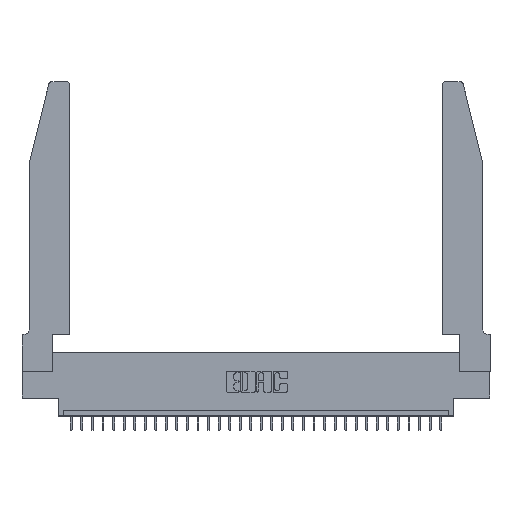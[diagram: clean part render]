
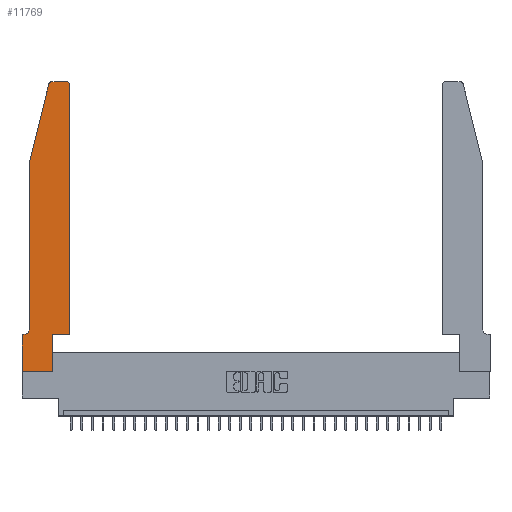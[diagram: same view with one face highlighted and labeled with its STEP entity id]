
A CAD part, top view. The second image highlights one B-rep face of the part: STEP entity #11769.
In plain terms, the highlighted planar face has unit normal (0, 0, 1).
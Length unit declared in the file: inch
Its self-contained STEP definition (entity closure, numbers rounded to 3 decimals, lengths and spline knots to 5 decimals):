
#304 = CARTESIAN_POINT ( 'NONE',  ( 0.284, 2.72, 0.37 ) ) ;
#1247 = PLANE ( 'NONE',  #5234 ) ;
#1288 = ORIENTED_EDGE ( 'NONE', *, *, #5457, .T. ) ;
#1545 = VERTEX_POINT ( 'NONE', #21221 ) ;
#2732 = ORIENTED_EDGE ( 'NONE', *, *, #26370, .T. ) ;
#2851 = LINE ( 'NONE', #30953, #15270 ) ;
#2899 = CARTESIAN_POINT ( 'NONE',  ( 0.4505, 0.35, 0.37 ) ) ;
#3214 = AXIS2_PLACEMENT_3D ( 'NONE', #30243, #17447, #30412 ) ;
#3261 = CARTESIAN_POINT ( 'NONE',  ( 0.2865, 0.35, 0.37 ) ) ;
#3734 = EDGE_CURVE ( 'NONE', #28187, #17740, #19510, .T. ) ;
#3958 = CARTESIAN_POINT ( 'NONE',  ( 0., 0., 0.37 ) ) ;
#4308 = VERTEX_POINT ( 'NONE', #21942 ) ;
#5141 = ORIENTED_EDGE ( 'NONE', *, *, #23761, .T. ) ;
#5234 = AXIS2_PLACEMENT_3D ( 'NONE', #29333, #29814, #16689 ) ;
#5243 = ORIENTED_EDGE ( 'NONE', *, *, #31368, .T. ) ;
#5287 = VERTEX_POINT ( 'NONE', #27833 ) ;
#5293 = DIRECTION ( 'NONE',  ( 0., 0., 1. ) ) ;
#5308 = EDGE_CURVE ( 'NONE', #10740, #15673, #17042, .T. ) ;
#5340 = LINE ( 'NONE', #24082, #5984 ) ;
#5457 = EDGE_CURVE ( 'NONE', #23564, #28187, #7693, .T. ) ;
#5984 = VECTOR ( 'NONE', #22964, 39.37008 ) ;
#6103 = CARTESIAN_POINT ( 'NONE',  ( 0.4205, 2.75, 0.37 ) ) ;
#6232 = DIRECTION ( 'NONE',  ( 0., 0., 1. ) ) ;
#6554 = FACE_OUTER_BOUND ( 'NONE', #18953, .T. ) ;
#6960 = VERTEX_POINT ( 'NONE', #25969 ) ;
#7246 = VECTOR ( 'NONE', #14596, 39.37008 ) ;
#7604 = EDGE_CURVE ( 'NONE', #17740, #6960, #30166, .T. ) ;
#7693 = LINE ( 'NONE', #18635, #9112 ) ;
#7771 = VECTOR ( 'NONE', #14862, 39.37008 ) ;
#8962 = EDGE_CURVE ( 'NONE', #14598, #28775, #19698, .T. ) ;
#9112 = VECTOR ( 'NONE', #27997, 39.37008 ) ;
#9160 = ORIENTED_EDGE ( 'NONE', *, *, #5308, .T. ) ;
#9676 = ORIENTED_EDGE ( 'NONE', *, *, #26531, .T. ) ;
#9686 = EDGE_CURVE ( 'NONE', #15673, #29340, #26753, .T. ) ;
#9692 = DIRECTION ( 'NONE',  ( -1., 0., 0. ) ) ;
#10474 = AXIS2_PLACEMENT_3D ( 'NONE', #304, #5293, #22910 ) ;
#10740 = VERTEX_POINT ( 'NONE', #30285 ) ;
#11769 = ADVANCED_FACE ( 'NONE', ( #6554 ), #1247, .T. ) ;
#12093 = CARTESIAN_POINT ( 'NONE',  ( 0.4505, 0.35, 0.37 ) ) ;
#12128 = EDGE_CURVE ( 'NONE', #4308, #23564, #15340, .T. ) ;
#12446 = ORIENTED_EDGE ( 'NONE', *, *, #25554, .T. ) ;
#13523 = CARTESIAN_POINT ( 'NONE',  ( 0.0055, 0.35, 0.37 ) ) ;
#14060 = ORIENTED_EDGE ( 'NONE', *, *, #9686, .T. ) ;
#14100 = ORIENTED_EDGE ( 'NONE', *, *, #7604, .T. ) ;
#14596 = DIRECTION ( 'NONE',  ( 1., 0., 0. ) ) ;
#14598 = VERTEX_POINT ( 'NONE', #13523 ) ;
#14621 = ORIENTED_EDGE ( 'NONE', *, *, #12128, .T. ) ;
#14859 = VECTOR ( 'NONE', #23164, 39.37008 ) ;
#14862 = DIRECTION ( 'NONE',  ( -0.239, -0.971, 0. ) ) ;
#15270 = VECTOR ( 'NONE', #23447, 39.37008 ) ;
#15340 = CIRCLE ( 'NONE', #32878, 0.03 ) ;
#15532 = LINE ( 'NONE', #2899, #14859 ) ;
#15673 = VERTEX_POINT ( 'NONE', #3261 ) ;
#16376 = DIRECTION ( 'NONE',  ( 1., 0., 0. ) ) ;
#16522 = CARTESIAN_POINT ( 'NONE',  ( 0.25487, 2.72718, 0.37 ) ) ;
#16689 = DIRECTION ( 'NONE',  ( 1., 0., 0. ) ) ;
#16748 = LINE ( 'NONE', #3958, #30800 ) ;
#17042 = LINE ( 'NONE', #25330, #31455 ) ;
#17447 = DIRECTION ( 'NONE',  ( 0., 0., -1. ) ) ;
#17526 = CIRCLE ( 'NONE', #3214, 0.07 ) ;
#17740 = VERTEX_POINT ( 'NONE', #16522 ) ;
#18635 = CARTESIAN_POINT ( 'NONE',  ( 0.2605, 2.75, 0.37 ) ) ;
#18953 = EDGE_LOOP ( 'NONE', ( #1288, #25549, #14100, #5243, #9676, #24670, #12446, #5141, #9160, #14060, #2732, #14621 ) ) ;
#19510 = CIRCLE ( 'NONE', #10474, 0.03 ) ;
#19698 = LINE ( 'NONE', #20004, #24824 ) ;
#20004 = CARTESIAN_POINT ( 'NONE',  ( 0.0755, 0.35, 0.37 ) ) ;
#21221 = CARTESIAN_POINT ( 'NONE',  ( 0.0755, 0.42, 0.37 ) ) ;
#21765 = CARTESIAN_POINT ( 'NONE',  ( 0., 0.35, 0.37 ) ) ;
#21942 = CARTESIAN_POINT ( 'NONE',  ( 0.4505, 2.72, 0.37 ) ) ;
#22667 = CARTESIAN_POINT ( 'NONE',  ( 0.0755, 2., 0.37 ) ) ;
#22910 = DIRECTION ( 'NONE',  ( 1., 0., 0. ) ) ;
#22964 = DIRECTION ( 'NONE',  ( 0., -1., 0. ) ) ;
#23164 = DIRECTION ( 'NONE',  ( 0., 1., 0. ) ) ;
#23447 = DIRECTION ( 'NONE',  ( 1., 0., 0. ) ) ;
#23564 = VERTEX_POINT ( 'NONE', #6103 ) ;
#23761 = EDGE_CURVE ( 'NONE', #5287, #10740, #2851, .T. ) ;
#24082 = CARTESIAN_POINT ( 'NONE',  ( 0.0755, 2., 0.37 ) ) ;
#24670 = ORIENTED_EDGE ( 'NONE', *, *, #8962, .T. ) ;
#24689 = DIRECTION ( 'NONE',  ( 0., 1., 0. ) ) ;
#24824 = VECTOR ( 'NONE', #9692, 39.37008 ) ;
#25330 = CARTESIAN_POINT ( 'NONE',  ( 0.2865, 0.35, 0.37 ) ) ;
#25549 = ORIENTED_EDGE ( 'NONE', *, *, #3734, .T. ) ;
#25554 = EDGE_CURVE ( 'NONE', #28775, #5287, #16748, .T. ) ;
#25969 = CARTESIAN_POINT ( 'NONE',  ( 0.0755, 2., 0.37 ) ) ;
#25989 = CARTESIAN_POINT ( 'NONE',  ( 0.284, 2.75, 0.37 ) ) ;
#26363 = CARTESIAN_POINT ( 'NONE',  ( 0.4505, 0.35, 0.37 ) ) ;
#26370 = EDGE_CURVE ( 'NONE', #29340, #4308, #15532, .T. ) ;
#26531 = EDGE_CURVE ( 'NONE', #1545, #14598, #17526, .T. ) ;
#26746 = DIRECTION ( 'NONE',  ( 0., -1., 0. ) ) ;
#26753 = LINE ( 'NONE', #12093, #7246 ) ;
#27833 = CARTESIAN_POINT ( 'NONE',  ( 0., 0., 0.37 ) ) ;
#27997 = DIRECTION ( 'NONE',  ( -1., 0., 0. ) ) ;
#28187 = VERTEX_POINT ( 'NONE', #25989 ) ;
#28775 = VERTEX_POINT ( 'NONE', #21765 ) ;
#29010 = CARTESIAN_POINT ( 'NONE',  ( 0.4205, 2.72, 0.37 ) ) ;
#29333 = CARTESIAN_POINT ( 'NONE',  ( 0., 0.35, 0.37 ) ) ;
#29340 = VERTEX_POINT ( 'NONE', #26363 ) ;
#29814 = DIRECTION ( 'NONE',  ( 0., 0., 1. ) ) ;
#30166 = LINE ( 'NONE', #22667, #7771 ) ;
#30243 = CARTESIAN_POINT ( 'NONE',  ( 0.0055, 0.42, 0.37 ) ) ;
#30285 = CARTESIAN_POINT ( 'NONE',  ( 0.2865, 0., 0.37 ) ) ;
#30412 = DIRECTION ( 'NONE',  ( -1., 0., 0. ) ) ;
#30800 = VECTOR ( 'NONE', #26746, 39.37008 ) ;
#30953 = CARTESIAN_POINT ( 'NONE',  ( 0., 0., 0.37 ) ) ;
#31368 = EDGE_CURVE ( 'NONE', #6960, #1545, #5340, .T. ) ;
#31455 = VECTOR ( 'NONE', #24689, 39.37008 ) ;
#32878 = AXIS2_PLACEMENT_3D ( 'NONE', #29010, #6232, #16376 ) ;
